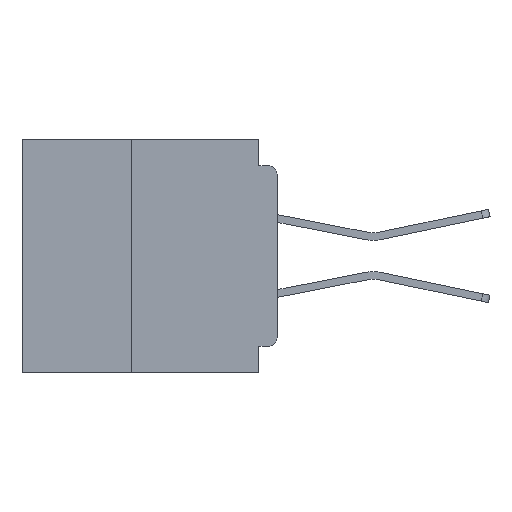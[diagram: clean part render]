
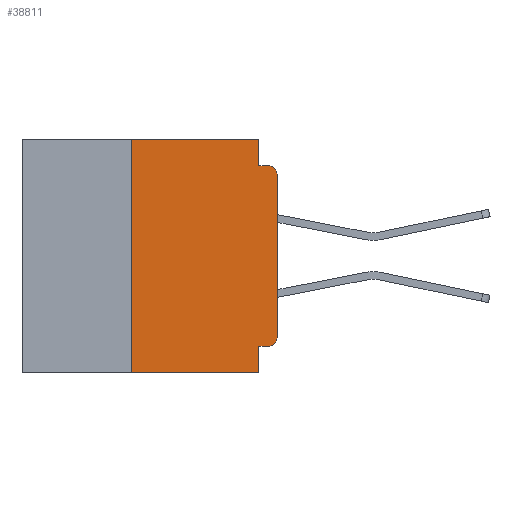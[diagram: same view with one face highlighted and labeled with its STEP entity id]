
A CAD part, left-side view. The second image highlights one B-rep face of the part: STEP entity #38811.
In plain terms, the highlighted planar face has unit normal (-1, 0, 0).
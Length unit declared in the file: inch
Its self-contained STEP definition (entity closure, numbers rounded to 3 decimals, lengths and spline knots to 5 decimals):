
#410 = CARTESIAN_POINT ( 'NONE',  ( 0., 0.015, -0.355 ) ) ;
#533 = ORIENTED_EDGE ( 'NONE', *, *, #14804, .F. ) ;
#1129 = ORIENTED_EDGE ( 'NONE', *, *, #15980, .F. ) ;
#1760 = LINE ( 'NONE', #16116, #10267 ) ;
#2106 = DIRECTION ( 'NONE',  ( -1., 0., 0. ) ) ;
#2798 = PLANE ( 'NONE',  #18749 ) ;
#3040 = VERTEX_POINT ( 'NONE', #38654 ) ;
#3052 = VECTOR ( 'NONE', #34668, 39.37008 ) ;
#4307 = ORIENTED_EDGE ( 'NONE', *, *, #22033, .F. ) ;
#4902 = VERTEX_POINT ( 'NONE', #18696 ) ;
#6491 = LINE ( 'NONE', #13210, #31972 ) ;
#6594 = VERTEX_POINT ( 'NONE', #37274 ) ;
#7103 = EDGE_CURVE ( 'NONE', #20515, #28901, #27449, .T. ) ;
#8785 = ORIENTED_EDGE ( 'NONE', *, *, #12472, .F. ) ;
#9134 = DIRECTION ( 'NONE',  ( 0., -1., 0. ) ) ;
#9285 = CARTESIAN_POINT ( 'NONE',  ( 0., 0.015, -0.34 ) ) ;
#9690 = DIRECTION ( 'NONE',  ( 0., 0., -1. ) ) ;
#10267 = VECTOR ( 'NONE', #19316, 39.37008 ) ;
#10694 = FACE_OUTER_BOUND ( 'NONE', #41396, .T. ) ;
#12472 = EDGE_CURVE ( 'NONE', #20515, #32016, #22237, .T. ) ;
#12499 = DIRECTION ( 'NONE',  ( 0., 0., -1. ) ) ;
#12925 = DIRECTION ( 'NONE',  ( 1., 0., 0. ) ) ;
#13210 = CARTESIAN_POINT ( 'NONE',  ( 0., 0., 0. ) ) ;
#14804 = EDGE_CURVE ( 'NONE', #30223, #3040, #20009, .T. ) ;
#14874 = VECTOR ( 'NONE', #9134, 39.37008 ) ;
#15575 = CARTESIAN_POINT ( 'NONE',  ( 0., 0., -0.045 ) ) ;
#15701 = VERTEX_POINT ( 'NONE', #20306 ) ;
#15871 = VECTOR ( 'NONE', #37392, 39.37008 ) ;
#15980 = EDGE_CURVE ( 'NONE', #3040, #6594, #41326, .T. ) ;
#16023 = CARTESIAN_POINT ( 'NONE',  ( 0., 0., -0.06 ) ) ;
#16084 = EDGE_CURVE ( 'NONE', #32016, #34829, #21351, .T. ) ;
#16116 = CARTESIAN_POINT ( 'NONE',  ( 0., 0.437, 0. ) ) ;
#16912 = CARTESIAN_POINT ( 'NONE',  ( 0., 0.031, -0.355 ) ) ;
#17234 = CARTESIAN_POINT ( 'NONE',  ( 0., 0., -0.34 ) ) ;
#18194 = VECTOR ( 'NONE', #28622, 39.37008 ) ;
#18696 = CARTESIAN_POINT ( 'NONE',  ( 0., 0.25, -0.4 ) ) ;
#18749 = AXIS2_PLACEMENT_3D ( 'NONE', #37806, #12925, #35267 ) ;
#19316 = DIRECTION ( 'NONE',  ( 0., -1., 0. ) ) ;
#20009 = LINE ( 'NONE', #31472, #3052 ) ;
#20306 = CARTESIAN_POINT ( 'NONE',  ( 0., 0.25, 0. ) ) ;
#20515 = VERTEX_POINT ( 'NONE', #410 ) ;
#20623 = ORIENTED_EDGE ( 'NONE', *, *, #21429, .T. ) ;
#21217 = CARTESIAN_POINT ( 'NONE',  ( 0., 0.015, -0.06 ) ) ;
#21343 = CARTESIAN_POINT ( 'NONE',  ( 0., 0.437, -0.4 ) ) ;
#21351 = LINE ( 'NONE', #25643, #36323 ) ;
#21429 = EDGE_CURVE ( 'NONE', #28901, #26010, #6491, .T. ) ;
#22030 = ORIENTED_EDGE ( 'NONE', *, *, #22649, .F. ) ;
#22033 = EDGE_CURVE ( 'NONE', #15701, #30223, #1760, .T. ) ;
#22237 = LINE ( 'NONE', #40096, #38190 ) ;
#22649 = EDGE_CURVE ( 'NONE', #4902, #15701, #35186, .T. ) ;
#23714 = ORIENTED_EDGE ( 'NONE', *, *, #36848, .T. ) ;
#24357 = LINE ( 'NONE', #21343, #15871 ) ;
#24449 = DIRECTION ( 'NONE',  ( 0., 0., -1. ) ) ;
#25447 = CARTESIAN_POINT ( 'NONE',  ( 0., 0.25, -0.4 ) ) ;
#25643 = CARTESIAN_POINT ( 'NONE',  ( 0., 0.031, -0.4 ) ) ;
#25956 = AXIS2_PLACEMENT_3D ( 'NONE', #9285, #31657, #12499 ) ;
#26010 = VERTEX_POINT ( 'NONE', #16023 ) ;
#27449 = CIRCLE ( 'NONE', #25956, 0.015 ) ;
#27907 = EDGE_CURVE ( 'NONE', #26010, #6594, #40247, .T. ) ;
#28622 = DIRECTION ( 'NONE',  ( 0., 0., 1. ) ) ;
#28901 = VERTEX_POINT ( 'NONE', #17234 ) ;
#29623 = CARTESIAN_POINT ( 'NONE',  ( 0., 0.031, 0. ) ) ;
#30223 = VERTEX_POINT ( 'NONE', #29623 ) ;
#31472 = CARTESIAN_POINT ( 'NONE',  ( 0., 0.031, 0. ) ) ;
#31530 = ORIENTED_EDGE ( 'NONE', *, *, #7103, .T. ) ;
#31657 = DIRECTION ( 'NONE',  ( -1., 0., 0. ) ) ;
#31972 = VECTOR ( 'NONE', #35553, 39.37008 ) ;
#32016 = VERTEX_POINT ( 'NONE', #16912 ) ;
#33181 = AXIS2_PLACEMENT_3D ( 'NONE', #21217, #2106, #24449 ) ;
#34547 = ORIENTED_EDGE ( 'NONE', *, *, #27907, .T. ) ;
#34668 = DIRECTION ( 'NONE',  ( 0., 0., -1. ) ) ;
#34829 = VERTEX_POINT ( 'NONE', #39793 ) ;
#35186 = LINE ( 'NONE', #25447, #18194 ) ;
#35267 = DIRECTION ( 'NONE',  ( 0., 0., -1. ) ) ;
#35553 = DIRECTION ( 'NONE',  ( 0., 0., 1. ) ) ;
#36323 = VECTOR ( 'NONE', #9690, 39.37008 ) ;
#36848 = EDGE_CURVE ( 'NONE', #4902, #34829, #24357, .T. ) ;
#36890 = DIRECTION ( 'NONE',  ( 0., 1., 0. ) ) ;
#37274 = CARTESIAN_POINT ( 'NONE',  ( 0., 0.015, -0.045 ) ) ;
#37392 = DIRECTION ( 'NONE',  ( 0., -1., 0. ) ) ;
#37806 = CARTESIAN_POINT ( 'NONE',  ( 0., 0.437, 0. ) ) ;
#38190 = VECTOR ( 'NONE', #36890, 39.37008 ) ;
#38654 = CARTESIAN_POINT ( 'NONE',  ( 0., 0.031, -0.045 ) ) ;
#38811 = ADVANCED_FACE ( 'NONE', ( #10694 ), #2798, .F. ) ;
#39571 = ORIENTED_EDGE ( 'NONE', *, *, #16084, .F. ) ;
#39793 = CARTESIAN_POINT ( 'NONE',  ( 0., 0.031, -0.4 ) ) ;
#40096 = CARTESIAN_POINT ( 'NONE',  ( 0., 0., -0.355 ) ) ;
#40247 = CIRCLE ( 'NONE', #33181, 0.015 ) ;
#41326 = LINE ( 'NONE', #15575, #14874 ) ;
#41396 = EDGE_LOOP ( 'NONE', ( #20623, #34547, #1129, #533, #4307, #22030, #23714, #39571, #8785, #31530 ) ) ;
